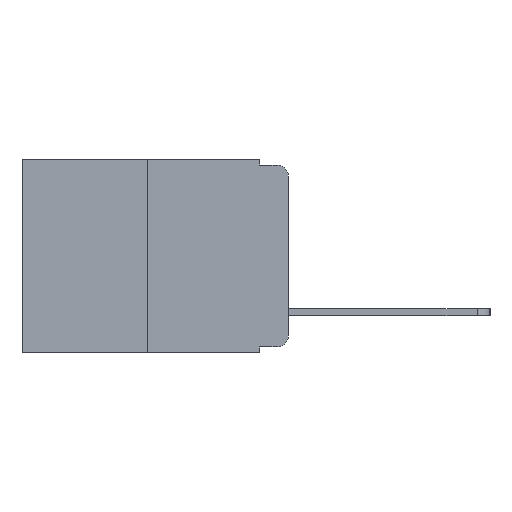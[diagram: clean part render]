
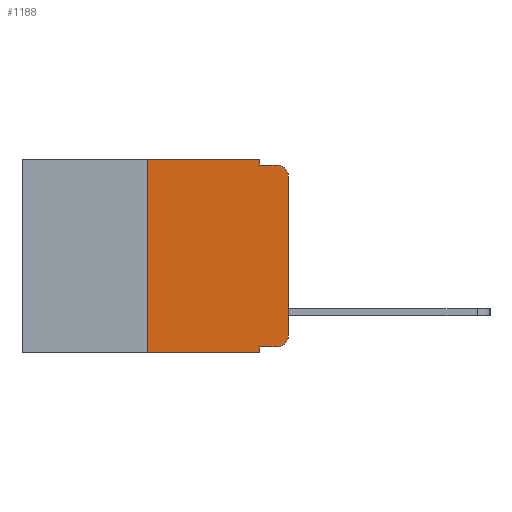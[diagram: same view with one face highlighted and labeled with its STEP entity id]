
A CAD part, left-side view. The second image highlights one B-rep face of the part: STEP entity #1188.
In plain terms, the highlighted planar face has unit normal (-1, 0, 0).
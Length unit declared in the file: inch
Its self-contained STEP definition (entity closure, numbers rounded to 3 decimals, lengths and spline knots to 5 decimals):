
#53 = VERTEX_POINT ( 'NONE', #3764 ) ;
#208 = VECTOR ( 'NONE', #7425, 39.37008 ) ;
#324 = PLANE ( 'NONE',  #9679 ) ;
#327 = CARTESIAN_POINT ( 'NONE',  ( 0., 0.473, 0. ) ) ;
#1125 = CARTESIAN_POINT ( 'NONE',  ( 0., 0., -0.313 ) ) ;
#1188 = ADVANCED_FACE ( 'NONE', ( #5385 ), #324, .F. ) ;
#1771 = CARTESIAN_POINT ( 'NONE',  ( 0., 0.051, -0.01 ) ) ;
#2309 = AXIS2_PLACEMENT_3D ( 'NONE', #13965, #4829, #15463 ) ;
#2875 = ORIENTED_EDGE ( 'NONE', *, *, #14525, .F. ) ;
#3163 = DIRECTION ( 'NONE',  ( 0., -1., 0. ) ) ;
#3275 = CIRCLE ( 'NONE', #10406, 0.02 ) ;
#3449 = LINE ( 'NONE', #16841, #11645 ) ;
#3764 = CARTESIAN_POINT ( 'NONE',  ( 0., 0.051, -0.333 ) ) ;
#3808 = VERTEX_POINT ( 'NONE', #10192 ) ;
#3959 = DIRECTION ( 'NONE',  ( 0., 0., -1. ) ) ;
#3981 = DIRECTION ( 'NONE',  ( 1., 0., 0. ) ) ;
#3983 = VECTOR ( 'NONE', #11431, 39.37008 ) ;
#4178 = CARTESIAN_POINT ( 'NONE',  ( 0., 0., 0. ) ) ;
#4494 = VECTOR ( 'NONE', #5727, 39.37008 ) ;
#4813 = VERTEX_POINT ( 'NONE', #19613 ) ;
#4826 = EDGE_LOOP ( 'NONE', ( #11815, #17128, #2875, #15526, #18046, #10195, #18457, #15565, #7324, #8176 ) ) ;
#4829 = DIRECTION ( 'NONE',  ( -1., 0., 0. ) ) ;
#5102 = VERTEX_POINT ( 'NONE', #17938 ) ;
#5385 = FACE_OUTER_BOUND ( 'NONE', #4826, .T. ) ;
#5408 = VECTOR ( 'NONE', #7543, 39.37008 ) ;
#5727 = DIRECTION ( 'NONE',  ( 0., 0., 1. ) ) ;
#5829 = VERTEX_POINT ( 'NONE', #13047 ) ;
#6375 = DIRECTION ( 'NONE',  ( -1., 0., 0. ) ) ;
#7324 = ORIENTED_EDGE ( 'NONE', *, *, #14940, .T. ) ;
#7425 = DIRECTION ( 'NONE',  ( 0., -1., 0. ) ) ;
#7543 = DIRECTION ( 'NONE',  ( 0., 0., 1. ) ) ;
#7604 = VECTOR ( 'NONE', #18166, 39.37008 ) ;
#7755 = CARTESIAN_POINT ( 'NONE',  ( 0., 0.051, 0. ) ) ;
#8176 = ORIENTED_EDGE ( 'NONE', *, *, #15003, .T. ) ;
#8598 = LINE ( 'NONE', #9000, #208 ) ;
#8855 = DIRECTION ( 'NONE',  ( 0., 0., -1. ) ) ;
#9000 = CARTESIAN_POINT ( 'NONE',  ( 0., 0.473, -0.343 ) ) ;
#9109 = VERTEX_POINT ( 'NONE', #18594 ) ;
#9679 = AXIS2_PLACEMENT_3D ( 'NONE', #327, #3981, #3959 ) ;
#10192 = CARTESIAN_POINT ( 'NONE',  ( 0., 0.25, 0. ) ) ;
#10195 = ORIENTED_EDGE ( 'NONE', *, *, #14849, .F. ) ;
#10200 = CARTESIAN_POINT ( 'NONE',  ( 0., 0.051, 0. ) ) ;
#10406 = AXIS2_PLACEMENT_3D ( 'NONE', #15487, #6375, #16961 ) ;
#10517 = LINE ( 'NONE', #15083, #5408 ) ;
#11431 = DIRECTION ( 'NONE',  ( 0., -1., 0. ) ) ;
#11645 = VECTOR ( 'NONE', #3163, 39.37008 ) ;
#11684 = LINE ( 'NONE', #7755, #7604 ) ;
#11815 = ORIENTED_EDGE ( 'NONE', *, *, #14162, .T. ) ;
#12169 = LINE ( 'NONE', #15281, #18946 ) ;
#12668 = LINE ( 'NONE', #4178, #4494 ) ;
#12910 = VERTEX_POINT ( 'NONE', #1771 ) ;
#13047 = CARTESIAN_POINT ( 'NONE',  ( 0., 0.051, -0.343 ) ) ;
#13104 = LINE ( 'NONE', #17325, #3983 ) ;
#13215 = VERTEX_POINT ( 'NONE', #13439 ) ;
#13439 = CARTESIAN_POINT ( 'NONE',  ( 0., 0.02, -0.01 ) ) ;
#13965 = CARTESIAN_POINT ( 'NONE',  ( 0., 0.02, -0.313 ) ) ;
#14101 = VERTEX_POINT ( 'NONE', #10200 ) ;
#14162 = EDGE_CURVE ( 'NONE', #17559, #9109, #12668, .T. ) ;
#14245 = CIRCLE ( 'NONE', #2309, 0.02 ) ;
#14363 = EDGE_CURVE ( 'NONE', #9109, #13215, #3275, .T. ) ;
#14525 = EDGE_CURVE ( 'NONE', #12910, #13215, #13104, .T. ) ;
#14746 = EDGE_CURVE ( 'NONE', #14101, #12910, #15853, .T. ) ;
#14849 = EDGE_CURVE ( 'NONE', #5102, #3808, #10517, .T. ) ;
#14932 = EDGE_CURVE ( 'NONE', #53, #5829, #11684, .T. ) ;
#14940 = EDGE_CURVE ( 'NONE', #53, #4813, #12169, .T. ) ;
#15003 = EDGE_CURVE ( 'NONE', #4813, #17559, #14245, .T. ) ;
#15083 = CARTESIAN_POINT ( 'NONE',  ( 0., 0.25, 0. ) ) ;
#15281 = CARTESIAN_POINT ( 'NONE',  ( 0., 0.051, -0.333 ) ) ;
#15410 = VECTOR ( 'NONE', #8855, 39.37008 ) ;
#15463 = DIRECTION ( 'NONE',  ( 0., 0., -1. ) ) ;
#15487 = CARTESIAN_POINT ( 'NONE',  ( 0., 0.02, -0.03 ) ) ;
#15526 = ORIENTED_EDGE ( 'NONE', *, *, #14746, .F. ) ;
#15565 = ORIENTED_EDGE ( 'NONE', *, *, #14932, .F. ) ;
#15675 = EDGE_CURVE ( 'NONE', #3808, #14101, #3449, .T. ) ;
#15853 = LINE ( 'NONE', #17742, #15410 ) ;
#16841 = CARTESIAN_POINT ( 'NONE',  ( 0., 0.473, 0. ) ) ;
#16961 = DIRECTION ( 'NONE',  ( 0., 0., -1. ) ) ;
#16972 = EDGE_CURVE ( 'NONE', #5102, #5829, #8598, .T. ) ;
#17128 = ORIENTED_EDGE ( 'NONE', *, *, #14363, .T. ) ;
#17325 = CARTESIAN_POINT ( 'NONE',  ( 0., 0.051, -0.01 ) ) ;
#17559 = VERTEX_POINT ( 'NONE', #1125 ) ;
#17742 = CARTESIAN_POINT ( 'NONE',  ( 0., 0.051, 0. ) ) ;
#17938 = CARTESIAN_POINT ( 'NONE',  ( 0., 0.25, -0.343 ) ) ;
#18046 = ORIENTED_EDGE ( 'NONE', *, *, #15675, .F. ) ;
#18099 = DIRECTION ( 'NONE',  ( 0., -1., 0. ) ) ;
#18166 = DIRECTION ( 'NONE',  ( 0., 0., -1. ) ) ;
#18457 = ORIENTED_EDGE ( 'NONE', *, *, #16972, .T. ) ;
#18594 = CARTESIAN_POINT ( 'NONE',  ( 0., 0., -0.03 ) ) ;
#18946 = VECTOR ( 'NONE', #18099, 39.37008 ) ;
#19613 = CARTESIAN_POINT ( 'NONE',  ( 0., 0.02, -0.333 ) ) ;
